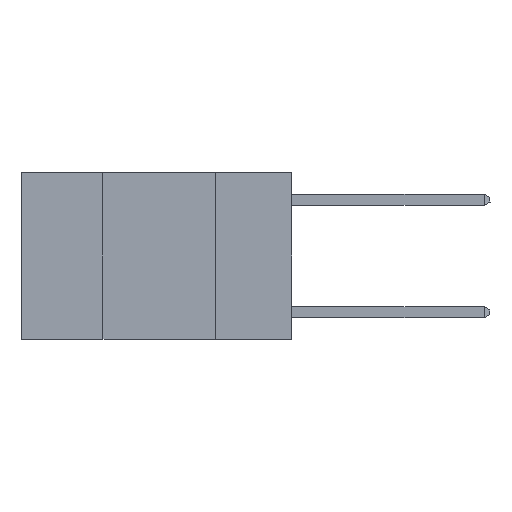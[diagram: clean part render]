
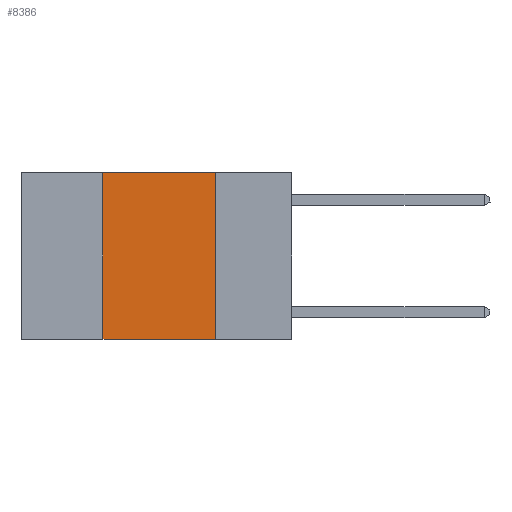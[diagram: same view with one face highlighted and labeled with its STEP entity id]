
A CAD part, left-side view. The second image highlights one B-rep face of the part: STEP entity #8386.
In plain terms, the highlighted planar face has unit normal (-1, 0, 0).
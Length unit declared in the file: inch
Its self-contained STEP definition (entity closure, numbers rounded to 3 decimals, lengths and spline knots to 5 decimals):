
#273 = CARTESIAN_POINT ( 'NONE',  ( 0., 0.6, 0. ) ) ;
#306 = ORIENTED_EDGE ( 'NONE', *, *, #13028, .F. ) ;
#371 = LINE ( 'NONE', #273, #7484 ) ;
#568 = ORIENTED_EDGE ( 'NONE', *, *, #13797, .F. ) ;
#1039 = VECTOR ( 'NONE', #5758, 39.37008 ) ;
#1463 = VERTEX_POINT ( 'NONE', #2436 ) ;
#2256 = DIRECTION ( 'NONE',  ( 1., 0., 0. ) ) ;
#2372 = EDGE_CURVE ( 'NONE', #1463, #3399, #16372, .T. ) ;
#2436 = CARTESIAN_POINT ( 'NONE',  ( 0., 0.42, -0.37 ) ) ;
#2889 = DIRECTION ( 'NONE',  ( 0., -1., 0. ) ) ;
#3399 = VERTEX_POINT ( 'NONE', #8479 ) ;
#3619 = DIRECTION ( 'NONE',  ( 0., 0., -1. ) ) ;
#3870 = FACE_OUTER_BOUND ( 'NONE', #7564, .T. ) ;
#3989 = CARTESIAN_POINT ( 'NONE',  ( 0., 0.6, -0.37 ) ) ;
#4113 = CARTESIAN_POINT ( 'NONE',  ( 0., 0.42, 0. ) ) ;
#4182 = ORIENTED_EDGE ( 'NONE', *, *, #7693, .F. ) ;
#4665 = VERTEX_POINT ( 'NONE', #17755 ) ;
#5758 = DIRECTION ( 'NONE',  ( 0., 0., 1. ) ) ;
#6185 = AXIS2_PLACEMENT_3D ( 'NONE', #6781, #2256, #3619 ) ;
#6781 = CARTESIAN_POINT ( 'NONE',  ( 0., 0.6, 0. ) ) ;
#7317 = VECTOR ( 'NONE', #9537, 39.37008 ) ;
#7484 = VECTOR ( 'NONE', #2889, 39.37008 ) ;
#7563 = LINE ( 'NONE', #11740, #12371 ) ;
#7564 = EDGE_LOOP ( 'NONE', ( #306, #568, #4182, #7749 ) ) ;
#7693 = EDGE_CURVE ( 'NONE', #1463, #9164, #11042, .T. ) ;
#7749 = ORIENTED_EDGE ( 'NONE', *, *, #2372, .T. ) ;
#8386 = ADVANCED_FACE ( 'NONE', ( #3870 ), #17781, .F. ) ;
#8479 = CARTESIAN_POINT ( 'NONE',  ( 0., 0.17, -0.37 ) ) ;
#9164 = VERTEX_POINT ( 'NONE', #11931 ) ;
#9537 = DIRECTION ( 'NONE',  ( 0., -1., 0. ) ) ;
#11042 = LINE ( 'NONE', #4113, #1039 ) ;
#11740 = CARTESIAN_POINT ( 'NONE',  ( 0., 0.17, 0. ) ) ;
#11931 = CARTESIAN_POINT ( 'NONE',  ( 0., 0.42, 0. ) ) ;
#12371 = VECTOR ( 'NONE', #13092, 39.37008 ) ;
#13028 = EDGE_CURVE ( 'NONE', #4665, #3399, #7563, .T. ) ;
#13092 = DIRECTION ( 'NONE',  ( 0., 0., -1. ) ) ;
#13797 = EDGE_CURVE ( 'NONE', #9164, #4665, #371, .T. ) ;
#16372 = LINE ( 'NONE', #3989, #7317 ) ;
#17755 = CARTESIAN_POINT ( 'NONE',  ( 0., 0.17, 0. ) ) ;
#17781 = PLANE ( 'NONE',  #6185 ) ;
